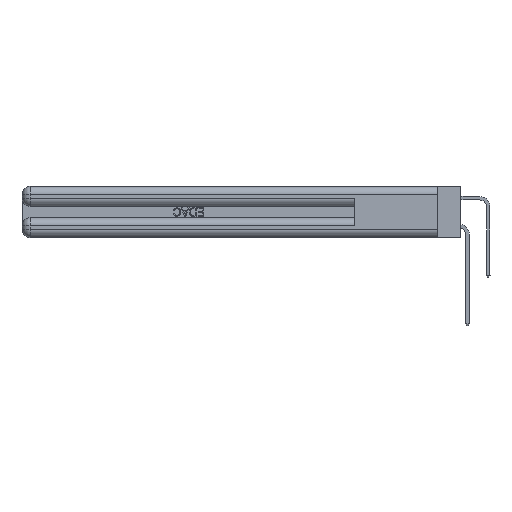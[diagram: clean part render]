
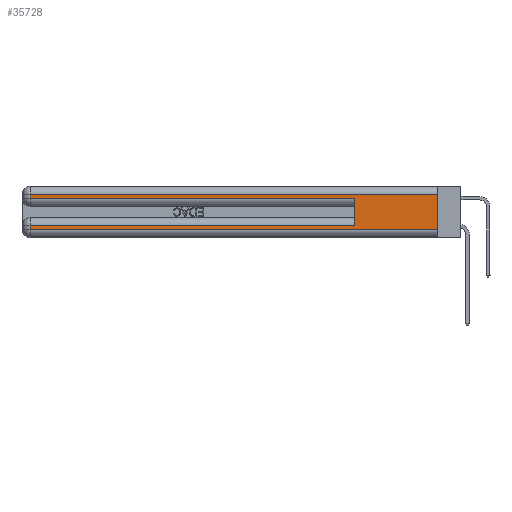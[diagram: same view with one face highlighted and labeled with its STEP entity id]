
A CAD part, left-side view. The second image highlights one B-rep face of the part: STEP entity #35728.
In plain terms, the highlighted planar face has unit normal (-1, 0, 0).
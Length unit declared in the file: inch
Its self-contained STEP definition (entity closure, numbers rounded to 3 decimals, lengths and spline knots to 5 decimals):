
#596 = VECTOR ( 'NONE', #5965, 39.37008 ) ;
#1126 = EDGE_CURVE ( 'NONE', #14373, #29241, #23554, .T. ) ;
#1786 = ORIENTED_EDGE ( 'NONE', *, *, #38823, .T. ) ;
#2532 = EDGE_CURVE ( 'NONE', #29241, #9089, #24003, .T. ) ;
#3025 = ORIENTED_EDGE ( 'NONE', *, *, #32849, .T. ) ;
#3221 = LINE ( 'NONE', #26727, #17908 ) ;
#4127 = ORIENTED_EDGE ( 'NONE', *, *, #38560, .T. ) ;
#4923 = DIRECTION ( 'NONE',  ( 0., -1., 0. ) ) ;
#5332 = CARTESIAN_POINT ( 'NONE',  ( 0., 0., 0.06 ) ) ;
#5373 = CARTESIAN_POINT ( 'NONE',  ( 0., 0., 0.31 ) ) ;
#5965 = DIRECTION ( 'NONE',  ( 0., 0., 1. ) ) ;
#6150 = CARTESIAN_POINT ( 'NONE',  ( 0., 0.6, 0.085 ) ) ;
#8340 = VECTOR ( 'NONE', #8356, 39.37008 ) ;
#8356 = DIRECTION ( 'NONE',  ( 0., 0., -1. ) ) ;
#8464 = ORIENTED_EDGE ( 'NONE', *, *, #40448, .F. ) ;
#8565 = DIRECTION ( 'NONE',  ( 1., 0., 0. ) ) ;
#9009 = LINE ( 'NONE', #40332, #596 ) ;
#9089 = VERTEX_POINT ( 'NONE', #38745 ) ;
#10096 = VERTEX_POINT ( 'NONE', #12789 ) ;
#10143 = ORIENTED_EDGE ( 'NONE', *, *, #26443, .F. ) ;
#10512 = CARTESIAN_POINT ( 'NONE',  ( 0., 0., 0.085 ) ) ;
#10865 = DIRECTION ( 'NONE',  ( 0., 0., -1. ) ) ;
#12114 = LINE ( 'NONE', #28693, #27794 ) ;
#12427 = CARTESIAN_POINT ( 'NONE',  ( 0., 2.94, 0.285 ) ) ;
#12652 = FACE_OUTER_BOUND ( 'NONE', #16951, .T. ) ;
#12789 = CARTESIAN_POINT ( 'NONE',  ( 0., 0.6, 0.285 ) ) ;
#12959 = DIRECTION ( 'NONE',  ( 0., 0., -1. ) ) ;
#14258 = VECTOR ( 'NONE', #29286, 39.37008 ) ;
#14372 = LINE ( 'NONE', #26462, #21675 ) ;
#14373 = VERTEX_POINT ( 'NONE', #6150 ) ;
#14379 = CARTESIAN_POINT ( 'NONE',  ( 0., 2.94, 0.37 ) ) ;
#15468 = CARTESIAN_POINT ( 'NONE',  ( 0., 0., 0.31 ) ) ;
#16802 = VERTEX_POINT ( 'NONE', #12427 ) ;
#16951 = EDGE_LOOP ( 'NONE', ( #10143, #3025, #21277, #4127, #8464, #31439, #24556, #1786 ) ) ;
#17820 = AXIS2_PLACEMENT_3D ( 'NONE', #30387, #8565, #30512 ) ;
#17908 = VECTOR ( 'NONE', #4923, 39.37008 ) ;
#17943 = DIRECTION ( 'NONE',  ( 0., 1., 0. ) ) ;
#18198 = VERTEX_POINT ( 'NONE', #15468 ) ;
#18865 = CARTESIAN_POINT ( 'NONE',  ( 0., 2.94, 0.085 ) ) ;
#21277 = ORIENTED_EDGE ( 'NONE', *, *, #23796, .T. ) ;
#21675 = VECTOR ( 'NONE', #10865, 39.37008 ) ;
#22789 = VERTEX_POINT ( 'NONE', #5332 ) ;
#23155 = VECTOR ( 'NONE', #17943, 39.37008 ) ;
#23554 = LINE ( 'NONE', #10512, #14258 ) ;
#23796 = EDGE_CURVE ( 'NONE', #34343, #16802, #23933, .T. ) ;
#23933 = LINE ( 'NONE', #28606, #31311 ) ;
#24003 = LINE ( 'NONE', #14379, #8340 ) ;
#24556 = ORIENTED_EDGE ( 'NONE', *, *, #2532, .T. ) ;
#26443 = EDGE_CURVE ( 'NONE', #18198, #22789, #14372, .T. ) ;
#26462 = CARTESIAN_POINT ( 'NONE',  ( 0., 0., 0.37 ) ) ;
#26727 = CARTESIAN_POINT ( 'NONE',  ( 0., 0., 0.06 ) ) ;
#27340 = PLANE ( 'NONE',  #17820 ) ;
#27794 = VECTOR ( 'NONE', #31834, 39.37008 ) ;
#28606 = CARTESIAN_POINT ( 'NONE',  ( 0., 2.94, 0.37 ) ) ;
#28693 = CARTESIAN_POINT ( 'NONE',  ( 0., 0., 0.285 ) ) ;
#29241 = VERTEX_POINT ( 'NONE', #18865 ) ;
#29286 = DIRECTION ( 'NONE',  ( 0., 1., 0. ) ) ;
#30387 = CARTESIAN_POINT ( 'NONE',  ( 0., 0., 0.37 ) ) ;
#30512 = DIRECTION ( 'NONE',  ( 0., 0., -1. ) ) ;
#31311 = VECTOR ( 'NONE', #12959, 39.37008 ) ;
#31439 = ORIENTED_EDGE ( 'NONE', *, *, #1126, .T. ) ;
#31526 = LINE ( 'NONE', #5373, #23155 ) ;
#31834 = DIRECTION ( 'NONE',  ( 0., -1., 0. ) ) ;
#32849 = EDGE_CURVE ( 'NONE', #18198, #34343, #31526, .T. ) ;
#34343 = VERTEX_POINT ( 'NONE', #35260 ) ;
#35260 = CARTESIAN_POINT ( 'NONE',  ( 0., 2.94, 0.31 ) ) ;
#35728 = ADVANCED_FACE ( 'NONE', ( #12652 ), #27340, .F. ) ;
#38560 = EDGE_CURVE ( 'NONE', #16802, #10096, #12114, .T. ) ;
#38745 = CARTESIAN_POINT ( 'NONE',  ( 0., 2.94, 0.06 ) ) ;
#38823 = EDGE_CURVE ( 'NONE', #9089, #22789, #3221, .T. ) ;
#40332 = CARTESIAN_POINT ( 'NONE',  ( 0., 0.6, 0.145 ) ) ;
#40448 = EDGE_CURVE ( 'NONE', #14373, #10096, #9009, .T. ) ;
